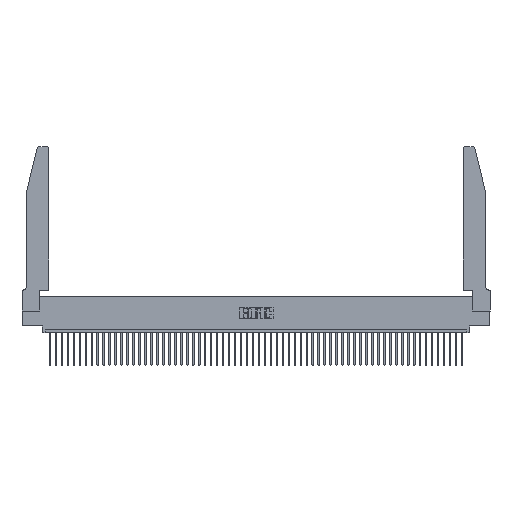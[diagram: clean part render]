
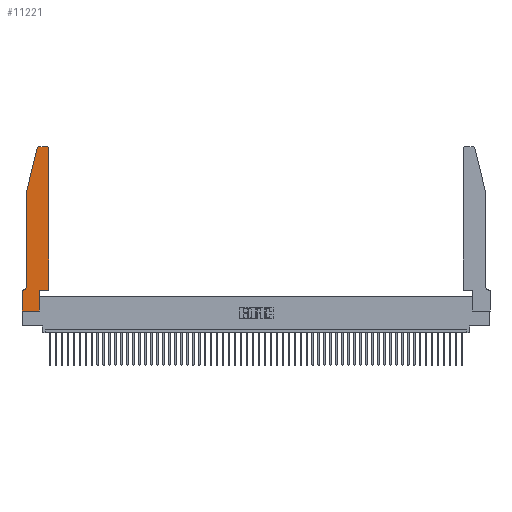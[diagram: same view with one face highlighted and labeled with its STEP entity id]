
A CAD part, top view. The second image highlights one B-rep face of the part: STEP entity #11221.
In plain terms, the highlighted planar face has unit normal (0, 0, 1).
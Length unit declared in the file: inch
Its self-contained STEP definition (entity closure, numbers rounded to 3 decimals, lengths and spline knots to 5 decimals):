
#1124 = CARTESIAN_POINT ( 'NONE',  ( 0., 0., 0.37 ) ) ;
#2016 = LINE ( 'NONE', #17315, #43563 ) ;
#2081 = CARTESIAN_POINT ( 'NONE',  ( 0.0755, 0.35, 0.37 ) ) ;
#3379 = EDGE_CURVE ( 'NONE', #5117, #8692, #44869, .T. ) ;
#3980 = VECTOR ( 'NONE', #51472, 39.37008 ) ;
#4104 = ORIENTED_EDGE ( 'NONE', *, *, #3379, .T. ) ;
#5005 = CARTESIAN_POINT ( 'NONE',  ( 0., 0.35, 0.37 ) ) ;
#5091 = DIRECTION ( 'NONE',  ( 0., -1., 0. ) ) ;
#5117 = VERTEX_POINT ( 'NONE', #27537 ) ;
#5315 = DIRECTION ( 'NONE',  ( 1., 0., 0. ) ) ;
#5330 = DIRECTION ( 'NONE',  ( 1., 0., 0. ) ) ;
#5470 = CARTESIAN_POINT ( 'NONE',  ( 0.0055, 0.35, 0.37 ) ) ;
#6360 = EDGE_CURVE ( 'NONE', #8692, #23838, #24096, .T. ) ;
#6374 = DIRECTION ( 'NONE',  ( 1., 0., 0. ) ) ;
#6657 = EDGE_CURVE ( 'NONE', #31999, #44111, #7199, .T. ) ;
#6844 = AXIS2_PLACEMENT_3D ( 'NONE', #17787, #21946, #5315 ) ;
#7058 = EDGE_CURVE ( 'NONE', #27861, #31615, #49400, .T. ) ;
#7181 = LINE ( 'NONE', #7318, #31903 ) ;
#7199 = LINE ( 'NONE', #48245, #3980 ) ;
#7318 = CARTESIAN_POINT ( 'NONE',  ( 0.2605, 2.75, 0.37 ) ) ;
#8343 = DIRECTION ( 'NONE',  ( 0., 1., 0. ) ) ;
#8692 = VERTEX_POINT ( 'NONE', #16183 ) ;
#8821 = CIRCLE ( 'NONE', #6844, 0.03 ) ;
#8942 = VERTEX_POINT ( 'NONE', #9026 ) ;
#9026 = CARTESIAN_POINT ( 'NONE',  ( 0.4205, 2.75, 0.37 ) ) ;
#9037 = VECTOR ( 'NONE', #28762, 39.37008 ) ;
#9252 = CARTESIAN_POINT ( 'NONE',  ( 0.0055, 0.42, 0.37 ) ) ;
#9287 = EDGE_CURVE ( 'NONE', #41342, #21424, #8821, .T. ) ;
#11062 = EDGE_CURVE ( 'NONE', #45903, #27861, #2016, .T. ) ;
#11221 = ADVANCED_FACE ( 'NONE', ( #19537 ), #19239, .T. ) ;
#11288 = CARTESIAN_POINT ( 'NONE',  ( 0.0755, 0.42, 0.37 ) ) ;
#11295 = DIRECTION ( 'NONE',  ( -0.239, -0.971, 0. ) ) ;
#12047 = CARTESIAN_POINT ( 'NONE',  ( 0.4505, 0.35, 0.37 ) ) ;
#12206 = CARTESIAN_POINT ( 'NONE',  ( 0.0755, 2., 0.37 ) ) ;
#13288 = DIRECTION ( 'NONE',  ( 0., 1., 0. ) ) ;
#15629 = ORIENTED_EDGE ( 'NONE', *, *, #24694, .T. ) ;
#16107 = ORIENTED_EDGE ( 'NONE', *, *, #9287, .T. ) ;
#16183 = CARTESIAN_POINT ( 'NONE',  ( 0.4505, 0.35, 0.37 ) ) ;
#17160 = DIRECTION ( 'NONE',  ( 0., -1., 0. ) ) ;
#17315 = CARTESIAN_POINT ( 'NONE',  ( 0.0755, 2., 0.37 ) ) ;
#17657 = EDGE_LOOP ( 'NONE', ( #15629, #16107, #51393, #22397, #27931, #36951, #26037, #30134, #49408, #4104, #18630, #22875 ) ) ;
#17787 = CARTESIAN_POINT ( 'NONE',  ( 0.284, 2.72, 0.37 ) ) ;
#18104 = LINE ( 'NONE', #21237, #50005 ) ;
#18617 = VERTEX_POINT ( 'NONE', #5005 ) ;
#18630 = ORIENTED_EDGE ( 'NONE', *, *, #6360, .T. ) ;
#19239 = PLANE ( 'NONE',  #32641 ) ;
#19537 = FACE_OUTER_BOUND ( 'NONE', #17657, .T. ) ;
#20250 = LINE ( 'NONE', #46138, #27384 ) ;
#20270 = EDGE_CURVE ( 'NONE', #31615, #18617, #30673, .T. ) ;
#21237 = CARTESIAN_POINT ( 'NONE',  ( 0., 0., 0.37 ) ) ;
#21424 = VERTEX_POINT ( 'NONE', #23462 ) ;
#21946 = DIRECTION ( 'NONE',  ( 0., 0., 1. ) ) ;
#22397 = ORIENTED_EDGE ( 'NONE', *, *, #11062, .T. ) ;
#22875 = ORIENTED_EDGE ( 'NONE', *, *, #39283, .T. ) ;
#23147 = EDGE_CURVE ( 'NONE', #44111, #5117, #20250, .T. ) ;
#23462 = CARTESIAN_POINT ( 'NONE',  ( 0.25487, 2.72718, 0.37 ) ) ;
#23818 = DIRECTION ( 'NONE',  ( -1., 0., 0. ) ) ;
#23838 = VERTEX_POINT ( 'NONE', #32077 ) ;
#24096 = LINE ( 'NONE', #49829, #33844 ) ;
#24694 = EDGE_CURVE ( 'NONE', #8942, #41342, #7181, .T. ) ;
#26037 = ORIENTED_EDGE ( 'NONE', *, *, #47970, .T. ) ;
#26712 = DIRECTION ( 'NONE',  ( -1., 0., 0. ) ) ;
#27384 = VECTOR ( 'NONE', #8343, 39.37008 ) ;
#27410 = CARTESIAN_POINT ( 'NONE',  ( 0., 0.35, 0.37 ) ) ;
#27537 = CARTESIAN_POINT ( 'NONE',  ( 0.2865, 0.35, 0.37 ) ) ;
#27861 = VERTEX_POINT ( 'NONE', #11288 ) ;
#27931 = ORIENTED_EDGE ( 'NONE', *, *, #7058, .T. ) ;
#28294 = AXIS2_PLACEMENT_3D ( 'NONE', #9252, #30157, #46365 ) ;
#28722 = VECTOR ( 'NONE', #11295, 39.37008 ) ;
#28762 = DIRECTION ( 'NONE',  ( 1., 0., 0. ) ) ;
#30134 = ORIENTED_EDGE ( 'NONE', *, *, #6657, .T. ) ;
#30157 = DIRECTION ( 'NONE',  ( 0., 0., -1. ) ) ;
#30673 = LINE ( 'NONE', #2081, #47553 ) ;
#31381 = CIRCLE ( 'NONE', #40076, 0.03 ) ;
#31479 = CARTESIAN_POINT ( 'NONE',  ( 0.2865, 0., 0.37 ) ) ;
#31615 = VERTEX_POINT ( 'NONE', #5470 ) ;
#31903 = VECTOR ( 'NONE', #23818, 39.37008 ) ;
#31999 = VERTEX_POINT ( 'NONE', #1124 ) ;
#32077 = CARTESIAN_POINT ( 'NONE',  ( 0.4505, 2.72, 0.37 ) ) ;
#32641 = AXIS2_PLACEMENT_3D ( 'NONE', #27410, #47765, #6374 ) ;
#33844 = VECTOR ( 'NONE', #13288, 39.37008 ) ;
#34378 = CARTESIAN_POINT ( 'NONE',  ( 0.4205, 2.72, 0.37 ) ) ;
#34552 = DIRECTION ( 'NONE',  ( 0., 0., 1. ) ) ;
#36231 = CARTESIAN_POINT ( 'NONE',  ( 0.0755, 2., 0.37 ) ) ;
#36951 = ORIENTED_EDGE ( 'NONE', *, *, #20270, .T. ) ;
#39283 = EDGE_CURVE ( 'NONE', #23838, #8942, #31381, .T. ) ;
#39572 = EDGE_CURVE ( 'NONE', #21424, #45903, #39746, .T. ) ;
#39746 = LINE ( 'NONE', #36231, #28722 ) ;
#39949 = CARTESIAN_POINT ( 'NONE',  ( 0.284, 2.75, 0.37 ) ) ;
#40076 = AXIS2_PLACEMENT_3D ( 'NONE', #34378, #34552, #5330 ) ;
#41342 = VERTEX_POINT ( 'NONE', #39949 ) ;
#43563 = VECTOR ( 'NONE', #17160, 39.37008 ) ;
#44111 = VERTEX_POINT ( 'NONE', #31479 ) ;
#44869 = LINE ( 'NONE', #12047, #9037 ) ;
#45903 = VERTEX_POINT ( 'NONE', #12206 ) ;
#46138 = CARTESIAN_POINT ( 'NONE',  ( 0.2865, 0.35, 0.37 ) ) ;
#46365 = DIRECTION ( 'NONE',  ( -1., 0., 0. ) ) ;
#47553 = VECTOR ( 'NONE', #26712, 39.37008 ) ;
#47765 = DIRECTION ( 'NONE',  ( 0., 0., 1. ) ) ;
#47970 = EDGE_CURVE ( 'NONE', #18617, #31999, #18104, .T. ) ;
#48245 = CARTESIAN_POINT ( 'NONE',  ( 0., 0., 0.37 ) ) ;
#49400 = CIRCLE ( 'NONE', #28294, 0.07 ) ;
#49408 = ORIENTED_EDGE ( 'NONE', *, *, #23147, .T. ) ;
#49829 = CARTESIAN_POINT ( 'NONE',  ( 0.4505, 0.35, 0.37 ) ) ;
#50005 = VECTOR ( 'NONE', #5091, 39.37008 ) ;
#51393 = ORIENTED_EDGE ( 'NONE', *, *, #39572, .T. ) ;
#51472 = DIRECTION ( 'NONE',  ( 1., 0., 0. ) ) ;
